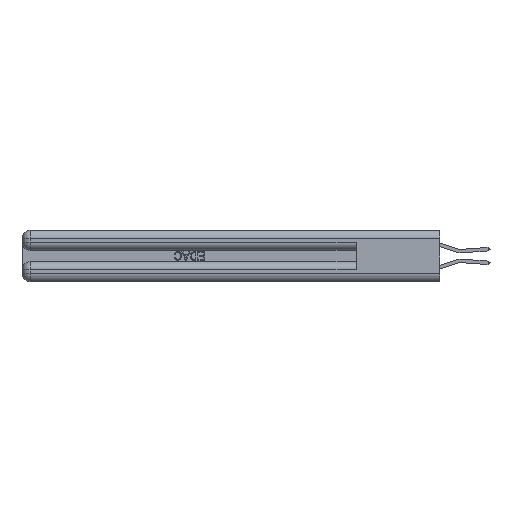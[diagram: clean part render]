
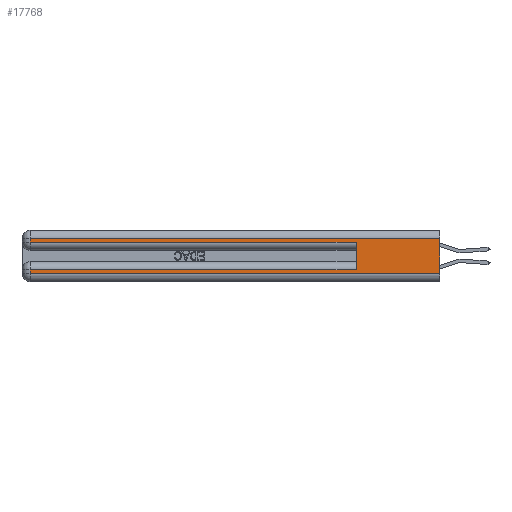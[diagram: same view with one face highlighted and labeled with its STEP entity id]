
A CAD part, left-side view. The second image highlights one B-rep face of the part: STEP entity #17768.
In plain terms, the highlighted planar face has unit normal (-1, 0, 0).
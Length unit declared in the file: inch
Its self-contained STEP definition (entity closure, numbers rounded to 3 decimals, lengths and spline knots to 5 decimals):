
#306 = EDGE_CURVE ( 'NONE', #43228, #35750, #41569, .T. ) ;
#3919 = DIRECTION ( 'NONE',  ( 0., 1., 0. ) ) ;
#4881 = EDGE_CURVE ( 'NONE', #17698, #34782, #30848, .T. ) ;
#5725 = VECTOR ( 'NONE', #21685, 39.37008 ) ;
#6336 = VECTOR ( 'NONE', #36740, 39.37008 ) ;
#6391 = ORIENTED_EDGE ( 'NONE', *, *, #27145, .T. ) ;
#6784 = LINE ( 'NONE', #7160, #23504 ) ;
#7160 = CARTESIAN_POINT ( 'NONE',  ( 0., 0.6, 0.145 ) ) ;
#8376 = VERTEX_POINT ( 'NONE', #16215 ) ;
#9529 = CARTESIAN_POINT ( 'NONE',  ( 0., 0., 0.285 ) ) ;
#9971 = CARTESIAN_POINT ( 'NONE',  ( 0., 0., 0.31 ) ) ;
#10853 = CARTESIAN_POINT ( 'NONE',  ( 0., 0., 0.06 ) ) ;
#11847 = ORIENTED_EDGE ( 'NONE', *, *, #28889, .T. ) ;
#12453 = EDGE_CURVE ( 'NONE', #17127, #34782, #32429, .T. ) ;
#12932 = EDGE_CURVE ( 'NONE', #8376, #39981, #25569, .T. ) ;
#13809 = VECTOR ( 'NONE', #39065, 39.37008 ) ;
#15743 = CARTESIAN_POINT ( 'NONE',  ( 0., 2.94, 0.06 ) ) ;
#16215 = CARTESIAN_POINT ( 'NONE',  ( 0., 2.94, 0.31 ) ) ;
#17127 = VERTEX_POINT ( 'NONE', #35985 ) ;
#17698 = VERTEX_POINT ( 'NONE', #15743 ) ;
#17768 = ADVANCED_FACE ( 'NONE', ( #18317 ), #32991, .F. ) ;
#18251 = EDGE_CURVE ( 'NONE', #43228, #33290, #6784, .T. ) ;
#18317 = FACE_OUTER_BOUND ( 'NONE', #25011, .T. ) ;
#19314 = VECTOR ( 'NONE', #34246, 39.37008 ) ;
#19732 = CARTESIAN_POINT ( 'NONE',  ( 0., 0.6, 0.285 ) ) ;
#19809 = ORIENTED_EDGE ( 'NONE', *, *, #306, .T. ) ;
#19948 = CARTESIAN_POINT ( 'NONE',  ( 0., 0., 0.37 ) ) ;
#20608 = ORIENTED_EDGE ( 'NONE', *, *, #12932, .T. ) ;
#21519 = ORIENTED_EDGE ( 'NONE', *, *, #18251, .F. ) ;
#21685 = DIRECTION ( 'NONE',  ( 0., 0., -1. ) ) ;
#22880 = DIRECTION ( 'NONE',  ( 0., 0., -1. ) ) ;
#23504 = VECTOR ( 'NONE', #30262, 39.37008 ) ;
#23704 = CARTESIAN_POINT ( 'NONE',  ( 0., 2.94, 0.37 ) ) ;
#25011 = EDGE_LOOP ( 'NONE', ( #26751, #6391, #20608, #11847, #21519, #19809, #33540, #36267 ) ) ;
#25515 = AXIS2_PLACEMENT_3D ( 'NONE', #19948, #36515, #22880 ) ;
#25569 = LINE ( 'NONE', #23704, #32372 ) ;
#26751 = ORIENTED_EDGE ( 'NONE', *, *, #12453, .F. ) ;
#26755 = LINE ( 'NONE', #39974, #6336 ) ;
#27145 = EDGE_CURVE ( 'NONE', #17127, #8376, #32646, .T. ) ;
#27254 = CARTESIAN_POINT ( 'NONE',  ( 0., 0., 0.06 ) ) ;
#28889 = EDGE_CURVE ( 'NONE', #39981, #33290, #35678, .T. ) ;
#30262 = DIRECTION ( 'NONE',  ( 0., 0., 1. ) ) ;
#30369 = CARTESIAN_POINT ( 'NONE',  ( 0., 2.94, 0.085 ) ) ;
#30423 = VECTOR ( 'NONE', #43200, 39.37008 ) ;
#30533 = VECTOR ( 'NONE', #3919, 39.37008 ) ;
#30848 = LINE ( 'NONE', #27254, #19314 ) ;
#31400 = CARTESIAN_POINT ( 'NONE',  ( 0., 2.94, 0.285 ) ) ;
#32372 = VECTOR ( 'NONE', #33382, 39.37008 ) ;
#32429 = LINE ( 'NONE', #34737, #5725 ) ;
#32646 = LINE ( 'NONE', #9971, #30533 ) ;
#32991 = PLANE ( 'NONE',  #25515 ) ;
#33290 = VERTEX_POINT ( 'NONE', #19732 ) ;
#33382 = DIRECTION ( 'NONE',  ( 0., 0., -1. ) ) ;
#33540 = ORIENTED_EDGE ( 'NONE', *, *, #36576, .T. ) ;
#34246 = DIRECTION ( 'NONE',  ( 0., -1., 0. ) ) ;
#34737 = CARTESIAN_POINT ( 'NONE',  ( 0., 0., 0.37 ) ) ;
#34782 = VERTEX_POINT ( 'NONE', #10853 ) ;
#35224 = CARTESIAN_POINT ( 'NONE',  ( 0., 0.6, 0.085 ) ) ;
#35678 = LINE ( 'NONE', #9529, #30423 ) ;
#35682 = CARTESIAN_POINT ( 'NONE',  ( 0., 0., 0.085 ) ) ;
#35750 = VERTEX_POINT ( 'NONE', #30369 ) ;
#35985 = CARTESIAN_POINT ( 'NONE',  ( 0., 0., 0.31 ) ) ;
#36267 = ORIENTED_EDGE ( 'NONE', *, *, #4881, .T. ) ;
#36515 = DIRECTION ( 'NONE',  ( 1., 0., 0. ) ) ;
#36576 = EDGE_CURVE ( 'NONE', #35750, #17698, #26755, .T. ) ;
#36740 = DIRECTION ( 'NONE',  ( 0., 0., -1. ) ) ;
#39065 = DIRECTION ( 'NONE',  ( 0., 1., 0. ) ) ;
#39974 = CARTESIAN_POINT ( 'NONE',  ( 0., 2.94, 0.37 ) ) ;
#39981 = VERTEX_POINT ( 'NONE', #31400 ) ;
#41569 = LINE ( 'NONE', #35682, #13809 ) ;
#43200 = DIRECTION ( 'NONE',  ( 0., -1., 0. ) ) ;
#43228 = VERTEX_POINT ( 'NONE', #35224 ) ;
